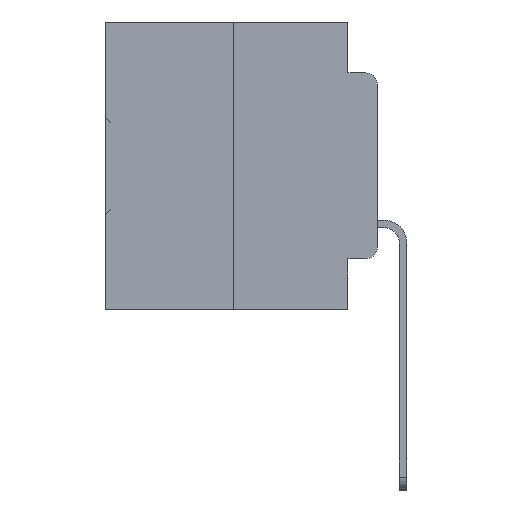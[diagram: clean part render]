
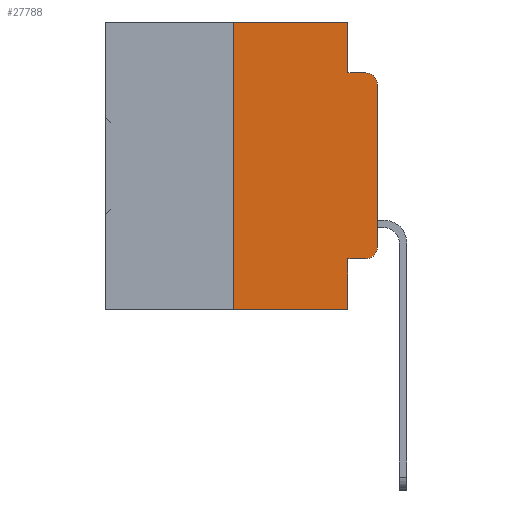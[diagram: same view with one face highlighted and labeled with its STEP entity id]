
A CAD part, left-side view. The second image highlights one B-rep face of the part: STEP entity #27788.
In plain terms, the highlighted planar face has unit normal (-1, 0, 0).
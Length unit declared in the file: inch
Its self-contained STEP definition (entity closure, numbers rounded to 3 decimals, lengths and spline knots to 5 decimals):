
#902 = ORIENTED_EDGE ( 'NONE', *, *, #19695, .F. ) ;
#912 = DIRECTION ( 'NONE',  ( 0., -1., 0. ) ) ;
#1726 = VECTOR ( 'NONE', #20627, 39.37008 ) ;
#1937 = ORIENTED_EDGE ( 'NONE', *, *, #28796, .T. ) ;
#2887 = ORIENTED_EDGE ( 'NONE', *, *, #20451, .T. ) ;
#3163 = CARTESIAN_POINT ( 'NONE',  ( 0., 0.051, 0. ) ) ;
#3607 = ORIENTED_EDGE ( 'NONE', *, *, #30135, .F. ) ;
#4335 = CARTESIAN_POINT ( 'NONE',  ( 0., 0., -0.3915 ) ) ;
#4654 = DIRECTION ( 'NONE',  ( 0., 0., -1. ) ) ;
#5060 = VERTEX_POINT ( 'NONE', #37617 ) ;
#5326 = DIRECTION ( 'NONE',  ( 0., -1., 0. ) ) ;
#6169 = CARTESIAN_POINT ( 'NONE',  ( 0., 0., 0. ) ) ;
#6453 = VECTOR ( 'NONE', #35199, 39.37008 ) ;
#6650 = CARTESIAN_POINT ( 'NONE',  ( 0., 0.473, -0.5 ) ) ;
#6792 = CIRCLE ( 'NONE', #36637, 0.02 ) ;
#6860 = CARTESIAN_POINT ( 'NONE',  ( 0., 0.051, -0.0885 ) ) ;
#6866 = FACE_OUTER_BOUND ( 'NONE', #16662, .T. ) ;
#7135 = EDGE_CURVE ( 'NONE', #19004, #19030, #8331, .T. ) ;
#7576 = LINE ( 'NONE', #8312, #29972 ) ;
#7585 = CARTESIAN_POINT ( 'NONE',  ( 0., 0.02, -0.1085 ) ) ;
#8263 = VECTOR ( 'NONE', #18029, 39.37008 ) ;
#8312 = CARTESIAN_POINT ( 'NONE',  ( 0., 0.25, 0. ) ) ;
#8331 = LINE ( 'NONE', #3163, #6453 ) ;
#10578 = DIRECTION ( 'NONE',  ( 0., 0., -1. ) ) ;
#11037 = CARTESIAN_POINT ( 'NONE',  ( 0., 0., -0.1085 ) ) ;
#11146 = EDGE_CURVE ( 'NONE', #19030, #15696, #19064, .T. ) ;
#11307 = VECTOR ( 'NONE', #912, 39.37008 ) ;
#11346 = CARTESIAN_POINT ( 'NONE',  ( 0., 0.051, 0. ) ) ;
#13090 = VECTOR ( 'NONE', #37335, 39.37008 ) ;
#13702 = VERTEX_POINT ( 'NONE', #22361 ) ;
#13933 = LINE ( 'NONE', #14904, #35213 ) ;
#14042 = ORIENTED_EDGE ( 'NONE', *, *, #11146, .F. ) ;
#14904 = CARTESIAN_POINT ( 'NONE',  ( 0., 0.051, -0.4115 ) ) ;
#14991 = ORIENTED_EDGE ( 'NONE', *, *, #15927, .F. ) ;
#15056 = EDGE_CURVE ( 'NONE', #18470, #15696, #6792, .T. ) ;
#15696 = VERTEX_POINT ( 'NONE', #19484 ) ;
#15927 = EDGE_CURVE ( 'NONE', #23236, #19004, #24765, .T. ) ;
#15967 = ORIENTED_EDGE ( 'NONE', *, *, #7135, .F. ) ;
#16034 = VECTOR ( 'NONE', #21469, 39.37008 ) ;
#16100 = DIRECTION ( 'NONE',  ( -1., 0., 0. ) ) ;
#16114 = LINE ( 'NONE', #6169, #8263 ) ;
#16170 = AXIS2_PLACEMENT_3D ( 'NONE', #33417, #16100, #36258 ) ;
#16537 = EDGE_CURVE ( 'NONE', #25279, #18965, #30633, .T. ) ;
#16662 = EDGE_LOOP ( 'NONE', ( #22420, #21453, #14042, #15967, #14991, #902, #1937, #3607, #2887, #20313 ) ) ;
#18029 = DIRECTION ( 'NONE',  ( 0., 0., 1. ) ) ;
#18470 = VERTEX_POINT ( 'NONE', #11037 ) ;
#18965 = VERTEX_POINT ( 'NONE', #4335 ) ;
#19004 = VERTEX_POINT ( 'NONE', #36515 ) ;
#19030 = VERTEX_POINT ( 'NONE', #28203 ) ;
#19064 = LINE ( 'NONE', #6860, #11307 ) ;
#19362 = CARTESIAN_POINT ( 'NONE',  ( 0., 0.473, 0. ) ) ;
#19484 = CARTESIAN_POINT ( 'NONE',  ( 0., 0.02, -0.0885 ) ) ;
#19695 = EDGE_CURVE ( 'NONE', #5060, #23236, #7576, .T. ) ;
#20313 = ORIENTED_EDGE ( 'NONE', *, *, #16537, .T. ) ;
#20423 = VERTEX_POINT ( 'NONE', #32128 ) ;
#20451 = EDGE_CURVE ( 'NONE', #20423, #25279, #13933, .T. ) ;
#20627 = DIRECTION ( 'NONE',  ( 0., -1., 0. ) ) ;
#20907 = LINE ( 'NONE', #11346, #13090 ) ;
#21399 = AXIS2_PLACEMENT_3D ( 'NONE', #19362, #22319, #4654 ) ;
#21453 = ORIENTED_EDGE ( 'NONE', *, *, #15056, .T. ) ;
#21469 = DIRECTION ( 'NONE',  ( 0., -1., 0. ) ) ;
#22319 = DIRECTION ( 'NONE',  ( 1., 0., 0. ) ) ;
#22361 = CARTESIAN_POINT ( 'NONE',  ( 0., 0.051, -0.5 ) ) ;
#22420 = ORIENTED_EDGE ( 'NONE', *, *, #22901, .T. ) ;
#22901 = EDGE_CURVE ( 'NONE', #18965, #18470, #16114, .T. ) ;
#23236 = VERTEX_POINT ( 'NONE', #36858 ) ;
#23803 = LINE ( 'NONE', #6650, #16034 ) ;
#24765 = LINE ( 'NONE', #26459, #1726 ) ;
#25279 = VERTEX_POINT ( 'NONE', #37450 ) ;
#25961 = DIRECTION ( 'NONE',  ( 0., 0., 1. ) ) ;
#26459 = CARTESIAN_POINT ( 'NONE',  ( 0., 0.473, 0. ) ) ;
#27788 = ADVANCED_FACE ( 'NONE', ( #6866 ), #36578, .F. ) ;
#28070 = DIRECTION ( 'NONE',  ( -1., 0., 0. ) ) ;
#28203 = CARTESIAN_POINT ( 'NONE',  ( 0., 0.051, -0.0885 ) ) ;
#28796 = EDGE_CURVE ( 'NONE', #5060, #13702, #23803, .T. ) ;
#29972 = VECTOR ( 'NONE', #25961, 39.37008 ) ;
#30135 = EDGE_CURVE ( 'NONE', #20423, #13702, #20907, .T. ) ;
#30633 = CIRCLE ( 'NONE', #16170, 0.02 ) ;
#32128 = CARTESIAN_POINT ( 'NONE',  ( 0., 0.051, -0.4115 ) ) ;
#33417 = CARTESIAN_POINT ( 'NONE',  ( 0., 0.02, -0.3915 ) ) ;
#35199 = DIRECTION ( 'NONE',  ( 0., 0., -1. ) ) ;
#35213 = VECTOR ( 'NONE', #5326, 39.37008 ) ;
#36258 = DIRECTION ( 'NONE',  ( 0., 0., -1. ) ) ;
#36515 = CARTESIAN_POINT ( 'NONE',  ( 0., 0.051, 0. ) ) ;
#36578 = PLANE ( 'NONE',  #21399 ) ;
#36637 = AXIS2_PLACEMENT_3D ( 'NONE', #7585, #28070, #10578 ) ;
#36858 = CARTESIAN_POINT ( 'NONE',  ( 0., 0.25, 0. ) ) ;
#37335 = DIRECTION ( 'NONE',  ( 0., 0., -1. ) ) ;
#37450 = CARTESIAN_POINT ( 'NONE',  ( 0., 0.02, -0.4115 ) ) ;
#37617 = CARTESIAN_POINT ( 'NONE',  ( 0., 0.25, -0.5 ) ) ;
